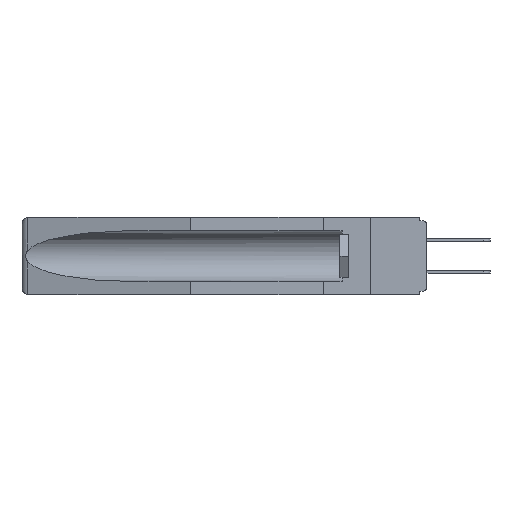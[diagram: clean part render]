
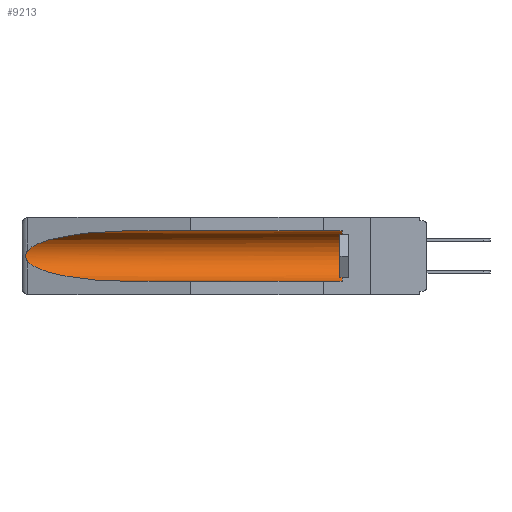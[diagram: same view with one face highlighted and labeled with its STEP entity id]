
A CAD part, left-side view. The second image highlights one B-rep face of the part: STEP entity #9213.
In plain terms, the highlighted cylindrical face has radius 2.857 mm (diameter 5.715 mm), a partial arc.
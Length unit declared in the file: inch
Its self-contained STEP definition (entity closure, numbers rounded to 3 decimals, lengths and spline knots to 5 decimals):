
#173 = VECTOR ( 'NONE', #11574, 39.37008 ) ;
#432 = LINE ( 'NONE', #17521, #16155 ) ;
#497 = B_SPLINE_CURVE_WITH_KNOTS ( 'NONE', 3,
 ( #936, #17360, #18587, #18764, #11475, #9939, #11408, #3817, #11212, #1054 ),
 .UNSPECIFIED., .F., .F.,
 ( 4, 2, 2, 2, 4 ),
 ( 0., 0.00029, 0.00058, 0.00087, 0.00117 ),
 .UNSPECIFIED. ) ;
#620 = CARTESIAN_POINT ( 'NONE',  ( 0.21114, 1.30732, -0.059 ) ) ;
#936 = CARTESIAN_POINT ( 'NONE',  ( 0.26537, 1.52718, -0.14972 ) ) ;
#1054 = CARTESIAN_POINT ( 'NONE',  ( 0.26537, 1.52718, -0.19328 ) ) ;
#1448 = CARTESIAN_POINT ( 'NONE',  ( 0.25451, 1.48313, -0.24835 ) ) ;
#1473 = CARTESIAN_POINT ( 'NONE',  ( 0.155, 1.07973, -0.059 ) ) ;
#2103 = ORIENTED_EDGE ( 'NONE', *, *, #3554, .T. ) ;
#3083 =( BOUNDED_CURVE ( )  B_SPLINE_CURVE ( 3, ( #13236, #1448, #10451, #17997 ),
 .UNSPECIFIED., .F., .F. ) 
 B_SPLINE_CURVE_WITH_KNOTS ( ( 4, 4 ),
 ( 0.1948, 1.5708 ),
 .UNSPECIFIED. ) 
 CURVE ( )  GEOMETRIC_REPRESENTATION_ITEM ( )  RATIONAL_B_SPLINE_CURVE ( ( 1., 0.848, 0.848, 1. ) ) 
 REPRESENTATION_ITEM ( '' )  );
#3222 = CARTESIAN_POINT ( 'NONE',  ( 0.26537, 1.52718, -0.14972 ) ) ;
#3248 = CARTESIAN_POINT ( 'NONE',  ( 0.26537, 1.52718, -0.14972 ) ) ;
#3554 = EDGE_CURVE ( 'NONE', #9728, #15272, #497, .T. ) ;
#3817 = CARTESIAN_POINT ( 'NONE',  ( 0.26655, 1.53094, -0.18657 ) ) ;
#4079 = LINE ( 'NONE', #11748, #173 ) ;
#4489 = ORIENTED_EDGE ( 'NONE', *, *, #10223, .T. ) ;
#4900 = DIRECTION ( 'NONE',  ( 0., 1., 0. ) ) ;
#5243 = AXIS2_PLACEMENT_3D ( 'NONE', #16605, #9061, #16676 ) ;
#5443 = ORIENTED_EDGE ( 'NONE', *, *, #9441, .T. ) ;
#5509 = CIRCLE ( 'NONE', #5243, 0.1125 ) ;
#5749 = DIRECTION ( 'NONE',  ( 0., 1., 0. ) ) ;
#6219 = CYLINDRICAL_SURFACE ( 'NONE', #7998, 0.1125 ) ;
#6439 = CARTESIAN_POINT ( 'NONE',  ( 0.155, 1.07973, -0.059 ) ) ;
#6558 = CARTESIAN_POINT ( 'NONE',  ( 0.155, -0.30754, -0.1715 ) ) ;
#7971 =( BOUNDED_CURVE ( )  B_SPLINE_CURVE ( 3, ( #6439, #620, #13852, #3248 ),
 .UNSPECIFIED., .F., .F. ) 
 B_SPLINE_CURVE_WITH_KNOTS ( ( 4, 4 ),
 ( 4.71239, 6.08839 ),
 .UNSPECIFIED. ) 
 CURVE ( )  GEOMETRIC_REPRESENTATION_ITEM ( )  RATIONAL_B_SPLINE_CURVE ( ( 1., 0.848, 0.848, 1. ) ) 
 REPRESENTATION_ITEM ( '' )  );
#7998 = AXIS2_PLACEMENT_3D ( 'NONE', #6558, #4900, #10455 ) ;
#8943 = CARTESIAN_POINT ( 'NONE',  ( 0.155, 1.07973, -0.284 ) ) ;
#9016 = FACE_OUTER_BOUND ( 'NONE', #17616, .T. ) ;
#9061 = DIRECTION ( 'NONE',  ( 0., -1., 0. ) ) ;
#9213 = ADVANCED_FACE ( 'NONE', ( #9016 ), #6219, .F. ) ;
#9336 = ORIENTED_EDGE ( 'NONE', *, *, #17489, .T. ) ;
#9441 = EDGE_CURVE ( 'NONE', #12186, #9728, #7971, .T. ) ;
#9728 = VERTEX_POINT ( 'NONE', #3222 ) ;
#9939 = CARTESIAN_POINT ( 'NONE',  ( 0.2675, 1.53308, -0.17534 ) ) ;
#9950 = CARTESIAN_POINT ( 'NONE',  ( 0.155, 0.126, -0.059 ) ) ;
#10071 = EDGE_CURVE ( 'NONE', #15928, #12767, #432, .T. ) ;
#10223 = EDGE_CURVE ( 'NONE', #15928, #11543, #5509, .T. ) ;
#10451 = CARTESIAN_POINT ( 'NONE',  ( 0.21114, 1.30732, -0.284 ) ) ;
#10455 = DIRECTION ( 'NONE',  ( 0., 0., 1. ) ) ;
#11119 = EDGE_CURVE ( 'NONE', #11543, #12186, #4079, .T. ) ;
#11212 = CARTESIAN_POINT ( 'NONE',  ( 0.26597, 1.5296, -0.19026 ) ) ;
#11408 = CARTESIAN_POINT ( 'NONE',  ( 0.2673, 1.53269, -0.17917 ) ) ;
#11475 = CARTESIAN_POINT ( 'NONE',  ( 0.2675, 1.53308, -0.16763 ) ) ;
#11543 = VERTEX_POINT ( 'NONE', #9950 ) ;
#11574 = DIRECTION ( 'NONE',  ( 0., 1., 0. ) ) ;
#11689 = CARTESIAN_POINT ( 'NONE',  ( 0.155, 0.126, -0.284 ) ) ;
#11748 = CARTESIAN_POINT ( 'NONE',  ( 0.155, -0.30754, -0.059 ) ) ;
#12186 = VERTEX_POINT ( 'NONE', #1473 ) ;
#12767 = VERTEX_POINT ( 'NONE', #8943 ) ;
#13236 = CARTESIAN_POINT ( 'NONE',  ( 0.26537, 1.52718, -0.19328 ) ) ;
#13852 = CARTESIAN_POINT ( 'NONE',  ( 0.25451, 1.48313, -0.09465 ) ) ;
#14549 = CARTESIAN_POINT ( 'NONE',  ( 0.26537, 1.52718, -0.19328 ) ) ;
#14760 = ORIENTED_EDGE ( 'NONE', *, *, #11119, .T. ) ;
#15272 = VERTEX_POINT ( 'NONE', #14549 ) ;
#15928 = VERTEX_POINT ( 'NONE', #11689 ) ;
#16155 = VECTOR ( 'NONE', #5749, 39.37008 ) ;
#16605 = CARTESIAN_POINT ( 'NONE',  ( 0.155, 0.126, -0.1715 ) ) ;
#16676 = DIRECTION ( 'NONE',  ( 0., 0., 1. ) ) ;
#17360 = CARTESIAN_POINT ( 'NONE',  ( 0.26597, 1.52961, -0.15275 ) ) ;
#17489 = EDGE_CURVE ( 'NONE', #15272, #12767, #3083, .T. ) ;
#17521 = CARTESIAN_POINT ( 'NONE',  ( 0.155, -0.30754, -0.284 ) ) ;
#17616 = EDGE_LOOP ( 'NONE', ( #5443, #2103, #9336, #18589, #4489, #14760 ) ) ;
#17997 = CARTESIAN_POINT ( 'NONE',  ( 0.155, 1.07973, -0.284 ) ) ;
#18587 = CARTESIAN_POINT ( 'NONE',  ( 0.26654, 1.53092, -0.15636 ) ) ;
#18589 = ORIENTED_EDGE ( 'NONE', *, *, #10071, .F. ) ;
#18764 = CARTESIAN_POINT ( 'NONE',  ( 0.2673, 1.5327, -0.16383 ) ) ;
